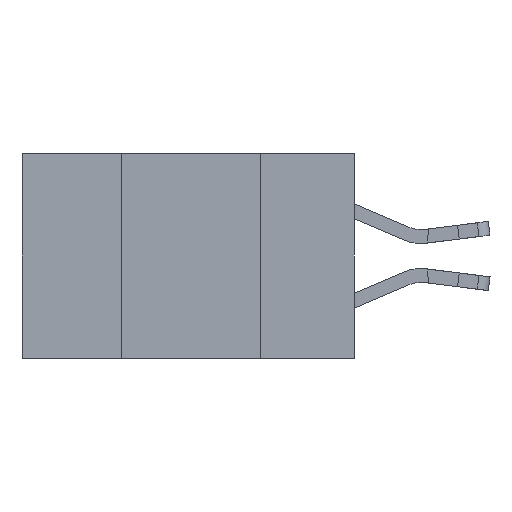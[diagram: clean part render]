
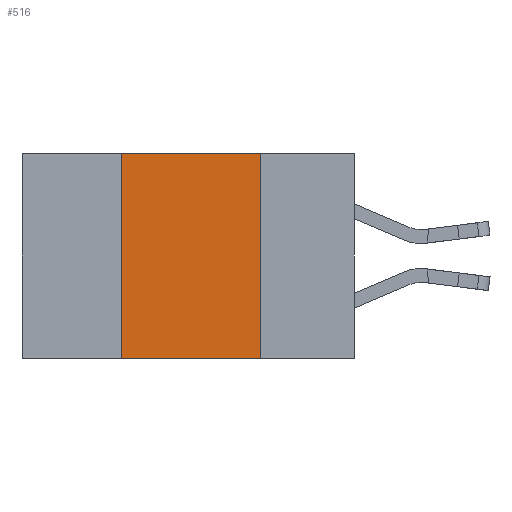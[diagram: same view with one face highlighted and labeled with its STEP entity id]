
A CAD part, left-side view. The second image highlights one B-rep face of the part: STEP entity #516.
In plain terms, the highlighted planar face has unit normal (-1, 0, 0).
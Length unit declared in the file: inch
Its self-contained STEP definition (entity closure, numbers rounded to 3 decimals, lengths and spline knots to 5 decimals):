
#137 = ORIENTED_EDGE ( 'NONE', *, *, #11801, .T. ) ;
#516 = ADVANCED_FACE ( 'NONE', ( #7225 ), #12226, .F. ) ;
#1088 = DIRECTION ( 'NONE',  ( 1., 0., 0. ) ) ;
#1963 = VECTOR ( 'NONE', #5885, 39.37008 ) ;
#2146 = LINE ( 'NONE', #11589, #11086 ) ;
#2896 = EDGE_CURVE ( 'NONE', #23422, #9811, #21567, .T. ) ;
#3777 = CARTESIAN_POINT ( 'NONE',  ( 0., 0.42, -0.37 ) ) ;
#5192 = CARTESIAN_POINT ( 'NONE',  ( 0., 0.6, 0. ) ) ;
#5885 = DIRECTION ( 'NONE',  ( 0., 0., 1. ) ) ;
#6426 = CARTESIAN_POINT ( 'NONE',  ( 0., 0.17, 0. ) ) ;
#7225 = FACE_OUTER_BOUND ( 'NONE', #10820, .T. ) ;
#7917 = DIRECTION ( 'NONE',  ( 0., -1., 0. ) ) ;
#9216 = ORIENTED_EDGE ( 'NONE', *, *, #2896, .F. ) ;
#9811 = VERTEX_POINT ( 'NONE', #6426 ) ;
#10820 = EDGE_LOOP ( 'NONE', ( #19125, #9216, #14275, #137 ) ) ;
#11086 = VECTOR ( 'NONE', #13527, 39.37008 ) ;
#11575 = VECTOR ( 'NONE', #15660, 39.37008 ) ;
#11589 = CARTESIAN_POINT ( 'NONE',  ( 0., 0.17, -0.37 ) ) ;
#11801 = EDGE_CURVE ( 'NONE', #12666, #17286, #17443, .T. ) ;
#11869 = VECTOR ( 'NONE', #7917, 39.37008 ) ;
#12120 = LINE ( 'NONE', #3777, #1963 ) ;
#12226 = PLANE ( 'NONE',  #22588 ) ;
#12666 = VERTEX_POINT ( 'NONE', #20058 ) ;
#13527 = DIRECTION ( 'NONE',  ( 0., 0., -1. ) ) ;
#14275 = ORIENTED_EDGE ( 'NONE', *, *, #20639, .F. ) ;
#14813 = DIRECTION ( 'NONE',  ( 0., 0., -1. ) ) ;
#15660 = DIRECTION ( 'NONE',  ( 0., -1., 0. ) ) ;
#16459 = CARTESIAN_POINT ( 'NONE',  ( 0., 0.6, 0. ) ) ;
#17271 = CARTESIAN_POINT ( 'NONE',  ( 0., 0.6, -0.37 ) ) ;
#17286 = VERTEX_POINT ( 'NONE', #22006 ) ;
#17443 = LINE ( 'NONE', #17271, #11869 ) ;
#19125 = ORIENTED_EDGE ( 'NONE', *, *, #21870, .F. ) ;
#20058 = CARTESIAN_POINT ( 'NONE',  ( 0., 0.42, -0.37 ) ) ;
#20639 = EDGE_CURVE ( 'NONE', #12666, #23422, #12120, .T. ) ;
#21567 = LINE ( 'NONE', #16459, #11575 ) ;
#21870 = EDGE_CURVE ( 'NONE', #9811, #17286, #2146, .T. ) ;
#22006 = CARTESIAN_POINT ( 'NONE',  ( 0., 0.17, -0.37 ) ) ;
#22588 = AXIS2_PLACEMENT_3D ( 'NONE', #5192, #1088, #14813 ) ;
#22960 = CARTESIAN_POINT ( 'NONE',  ( 0., 0.42, 0. ) ) ;
#23422 = VERTEX_POINT ( 'NONE', #22960 ) ;
